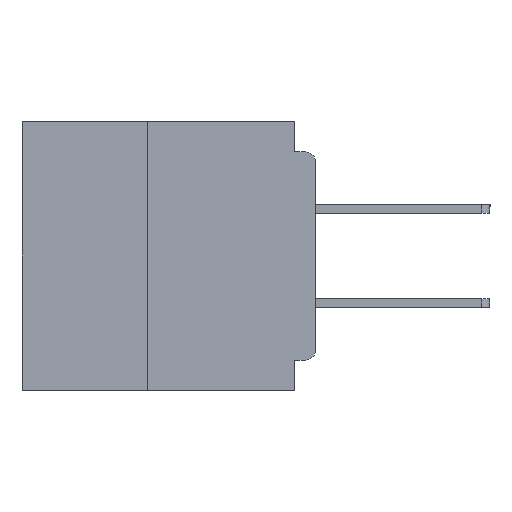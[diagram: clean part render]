
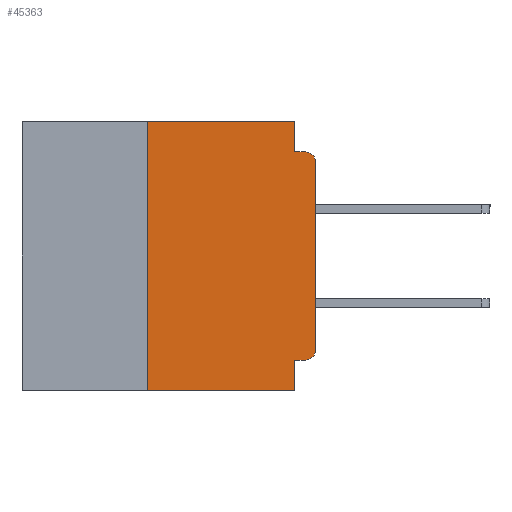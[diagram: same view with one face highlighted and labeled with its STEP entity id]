
A CAD part, left-side view. The second image highlights one B-rep face of the part: STEP entity #45363.
In plain terms, the highlighted planar face has unit normal (-1, 0, 0).
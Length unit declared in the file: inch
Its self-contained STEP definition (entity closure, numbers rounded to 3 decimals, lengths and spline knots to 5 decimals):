
#3876 = VERTEX_POINT ( 'NONE', #11687 ) ;
#3972 = DIRECTION ( 'NONE',  ( 0., 0., -1. ) ) ;
#3977 = ORIENTED_EDGE ( 'NONE', *, *, #42293, .F. ) ;
#4025 = AXIS2_PLACEMENT_3D ( 'NONE', #28931, #4337, #33043 ) ;
#4337 = DIRECTION ( 'NONE',  ( -1., 0., 0. ) ) ;
#5123 = ORIENTED_EDGE ( 'NONE', *, *, #42679, .T. ) ;
#5717 = VECTOR ( 'NONE', #26022, 39.37008 ) ;
#5898 = VECTOR ( 'NONE', #45551, 39.37008 ) ;
#6442 = AXIS2_PLACEMENT_3D ( 'NONE', #38003, #13476, #42130 ) ;
#7148 = CARTESIAN_POINT ( 'NONE',  ( 0., 0., -0.34 ) ) ;
#7170 = ORIENTED_EDGE ( 'NONE', *, *, #12828, .F. ) ;
#7187 = DIRECTION ( 'NONE',  ( 0., 0., 1. ) ) ;
#9004 = LINE ( 'NONE', #16969, #40490 ) ;
#11415 = FACE_OUTER_BOUND ( 'NONE', #24325, .T. ) ;
#11555 = VECTOR ( 'NONE', #7187, 39.37008 ) ;
#11687 = CARTESIAN_POINT ( 'NONE',  ( 0., 0.031, -0.045 ) ) ;
#11768 = VERTEX_POINT ( 'NONE', #33347 ) ;
#12828 = EDGE_CURVE ( 'NONE', #3876, #24562, #16502, .T. ) ;
#13476 = DIRECTION ( 'NONE',  ( 1., 0., 0. ) ) ;
#14819 = VERTEX_POINT ( 'NONE', #49520 ) ;
#15018 = ORIENTED_EDGE ( 'NONE', *, *, #44178, .F. ) ;
#15529 = EDGE_CURVE ( 'NONE', #49475, #47741, #37223, .T. ) ;
#16502 = LINE ( 'NONE', #52931, #39586 ) ;
#16969 = CARTESIAN_POINT ( 'NONE',  ( 0., 0.031, 0. ) ) ;
#18443 = CIRCLE ( 'NONE', #4025, 0.015 ) ;
#19123 = LINE ( 'NONE', #48349, #50593 ) ;
#19283 = CARTESIAN_POINT ( 'NONE',  ( 0., 0., -0.355 ) ) ;
#20450 = VERTEX_POINT ( 'NONE', #27492 ) ;
#21079 = DIRECTION ( 'NONE',  ( 0., 0., -1. ) ) ;
#22457 = LINE ( 'NONE', #48154, #11555 ) ;
#22995 = LINE ( 'NONE', #19283, #35180 ) ;
#23363 = DIRECTION ( 'NONE',  ( 0., 1., 0. ) ) ;
#23612 = EDGE_CURVE ( 'NONE', #14819, #49475, #22995, .T. ) ;
#24142 = DIRECTION ( 'NONE',  ( 0., -1., 0. ) ) ;
#24325 = EDGE_LOOP ( 'NONE', ( #5123, #53414, #7170, #3977, #15018, #29672, #44550, #35521, #28453, #48459 ) ) ;
#24562 = VERTEX_POINT ( 'NONE', #49712 ) ;
#25580 = PLANE ( 'NONE',  #6442 ) ;
#26022 = DIRECTION ( 'NONE',  ( 0., 0., -1. ) ) ;
#26906 = LINE ( 'NONE', #42235, #36588 ) ;
#27492 = CARTESIAN_POINT ( 'NONE',  ( 0., 0.25, -0.4 ) ) ;
#28453 = ORIENTED_EDGE ( 'NONE', *, *, #23612, .F. ) ;
#28455 = CARTESIAN_POINT ( 'NONE',  ( 0., 0.031, 0. ) ) ;
#28571 = DIRECTION ( 'NONE',  ( -1., 0., 0. ) ) ;
#28931 = CARTESIAN_POINT ( 'NONE',  ( 0., 0.015, -0.06 ) ) ;
#29002 = LINE ( 'NONE', #41408, #5898 ) ;
#29133 = VERTEX_POINT ( 'NONE', #28455 ) ;
#29672 = ORIENTED_EDGE ( 'NONE', *, *, #36531, .F. ) ;
#29830 = CIRCLE ( 'NONE', #52314, 0.015 ) ;
#33043 = DIRECTION ( 'NONE',  ( 0., 0., -1. ) ) ;
#33347 = CARTESIAN_POINT ( 'NONE',  ( 0., 0., -0.06 ) ) ;
#34492 = VERTEX_POINT ( 'NONE', #7148 ) ;
#35180 = VECTOR ( 'NONE', #23363, 39.37008 ) ;
#35521 = ORIENTED_EDGE ( 'NONE', *, *, #15529, .F. ) ;
#36083 = CARTESIAN_POINT ( 'NONE',  ( 0., 0.031, -0.4 ) ) ;
#36531 = EDGE_CURVE ( 'NONE', #20450, #51456, #29002, .T. ) ;
#36588 = VECTOR ( 'NONE', #38272, 39.37008 ) ;
#37223 = LINE ( 'NONE', #50709, #5717 ) ;
#38003 = CARTESIAN_POINT ( 'NONE',  ( 0., 0.437, 0. ) ) ;
#38272 = DIRECTION ( 'NONE',  ( 0., -1., 0. ) ) ;
#39586 = VECTOR ( 'NONE', #24142, 39.37008 ) ;
#40435 = CARTESIAN_POINT ( 'NONE',  ( 0., 0.031, -0.355 ) ) ;
#40490 = VECTOR ( 'NONE', #21079, 39.37008 ) ;
#41408 = CARTESIAN_POINT ( 'NONE',  ( 0., 0.25, -0.4 ) ) ;
#41670 = CARTESIAN_POINT ( 'NONE',  ( 0., 0.25, 0. ) ) ;
#42130 = DIRECTION ( 'NONE',  ( 0., 0., -1. ) ) ;
#42235 = CARTESIAN_POINT ( 'NONE',  ( 0., 0.437, 0. ) ) ;
#42293 = EDGE_CURVE ( 'NONE', #29133, #3876, #9004, .T. ) ;
#42679 = EDGE_CURVE ( 'NONE', #34492, #11768, #22457, .T. ) ;
#44178 = EDGE_CURVE ( 'NONE', #51456, #29133, #26906, .T. ) ;
#44550 = ORIENTED_EDGE ( 'NONE', *, *, #46308, .T. ) ;
#45363 = ADVANCED_FACE ( 'NONE', ( #11415 ), #25580, .F. ) ;
#45551 = DIRECTION ( 'NONE',  ( 0., 0., 1. ) ) ;
#45876 = EDGE_CURVE ( 'NONE', #11768, #24562, #18443, .T. ) ;
#46308 = EDGE_CURVE ( 'NONE', #20450, #47741, #19123, .T. ) ;
#47193 = EDGE_CURVE ( 'NONE', #14819, #34492, #29830, .T. ) ;
#47741 = VERTEX_POINT ( 'NONE', #36083 ) ;
#48154 = CARTESIAN_POINT ( 'NONE',  ( 0., 0., 0. ) ) ;
#48349 = CARTESIAN_POINT ( 'NONE',  ( 0., 0.437, -0.4 ) ) ;
#48459 = ORIENTED_EDGE ( 'NONE', *, *, #47193, .T. ) ;
#49475 = VERTEX_POINT ( 'NONE', #40435 ) ;
#49520 = CARTESIAN_POINT ( 'NONE',  ( 0., 0.015, -0.355 ) ) ;
#49712 = CARTESIAN_POINT ( 'NONE',  ( 0., 0.015, -0.045 ) ) ;
#50593 = VECTOR ( 'NONE', #52481, 39.37008 ) ;
#50709 = CARTESIAN_POINT ( 'NONE',  ( 0., 0.031, -0.4 ) ) ;
#51456 = VERTEX_POINT ( 'NONE', #41670 ) ;
#52314 = AXIS2_PLACEMENT_3D ( 'NONE', #53257, #28571, #3972 ) ;
#52481 = DIRECTION ( 'NONE',  ( 0., -1., 0. ) ) ;
#52931 = CARTESIAN_POINT ( 'NONE',  ( 0., 0., -0.045 ) ) ;
#53257 = CARTESIAN_POINT ( 'NONE',  ( 0., 0.015, -0.34 ) ) ;
#53414 = ORIENTED_EDGE ( 'NONE', *, *, #45876, .T. ) ;
